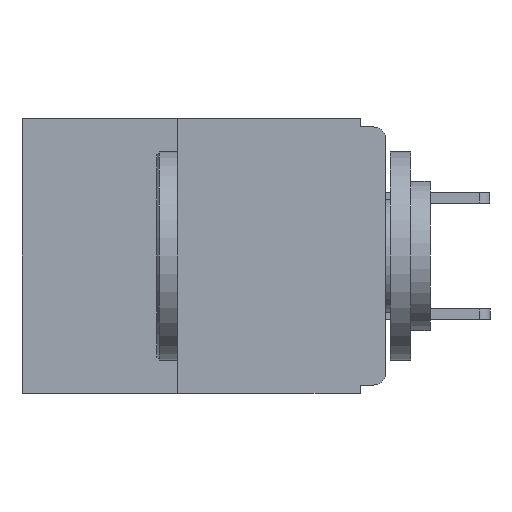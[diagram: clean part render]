
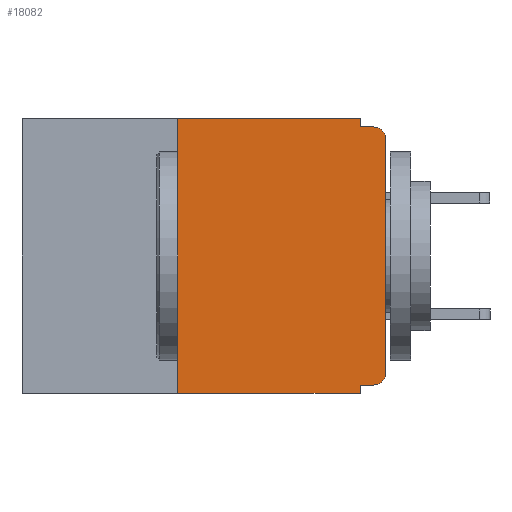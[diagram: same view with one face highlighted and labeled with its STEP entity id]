
A CAD part, left-side view. The second image highlights one B-rep face of the part: STEP entity #18082.
In plain terms, the highlighted planar face has unit normal (-1, 0, 0).
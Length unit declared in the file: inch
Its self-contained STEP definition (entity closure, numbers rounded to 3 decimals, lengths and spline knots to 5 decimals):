
#1279 = VERTEX_POINT ( 'NONE', #4539 ) ;
#1615 = DIRECTION ( 'NONE',  ( 0., 0., -1. ) ) ;
#1627 = AXIS2_PLACEMENT_3D ( 'NONE', #28823, #14491, #31188 ) ;
#1964 = EDGE_CURVE ( 'NONE', #20621, #14345, #23532, .T. ) ;
#3855 = VECTOR ( 'NONE', #27006, 39.37008 ) ;
#4539 = CARTESIAN_POINT ( 'NONE',  ( 0., 0.031, -0.32 ) ) ;
#4628 = DIRECTION ( 'NONE',  ( 0., 1., 0. ) ) ;
#4742 = CARTESIAN_POINT ( 'NONE',  ( 0., 0., -0.32 ) ) ;
#4743 = EDGE_CURVE ( 'NONE', #6605, #1279, #22581, .T. ) ;
#5766 = CARTESIAN_POINT ( 'NONE',  ( 0., 0.437, -0.33 ) ) ;
#5792 = VERTEX_POINT ( 'NONE', #30794 ) ;
#6011 = EDGE_CURVE ( 'NONE', #9688, #10685, #11187, .T. ) ;
#6605 = VERTEX_POINT ( 'NONE', #19673 ) ;
#6651 = DIRECTION ( 'NONE',  ( 0., 0., -1. ) ) ;
#6669 = CIRCLE ( 'NONE', #23854, 0.015 ) ;
#6970 = LINE ( 'NONE', #5766, #31062 ) ;
#7054 = CARTESIAN_POINT ( 'NONE',  ( 0., 0.015, -0.305 ) ) ;
#7147 = ORIENTED_EDGE ( 'NONE', *, *, #6011, .F. ) ;
#7919 = ORIENTED_EDGE ( 'NONE', *, *, #16331, .T. ) ;
#8167 = ORIENTED_EDGE ( 'NONE', *, *, #14884, .T. ) ;
#8579 = ORIENTED_EDGE ( 'NONE', *, *, #21228, .T. ) ;
#8981 = VECTOR ( 'NONE', #4628, 39.37008 ) ;
#9004 = CARTESIAN_POINT ( 'NONE',  ( 0., 0., 0. ) ) ;
#9572 = DIRECTION ( 'NONE',  ( 0., 0., -1. ) ) ;
#9688 = VERTEX_POINT ( 'NONE', #27475 ) ;
#10685 = VERTEX_POINT ( 'NONE', #12097 ) ;
#11022 = EDGE_CURVE ( 'NONE', #5792, #10685, #27361, .T. ) ;
#11187 = LINE ( 'NONE', #27444, #3855 ) ;
#11451 = VECTOR ( 'NONE', #17022, 39.37008 ) ;
#12097 = CARTESIAN_POINT ( 'NONE',  ( 0., 0.015, -0.01 ) ) ;
#12855 = LINE ( 'NONE', #25649, #31166 ) ;
#12887 = CARTESIAN_POINT ( 'NONE',  ( 0., 0.25, -0.33 ) ) ;
#13094 = ORIENTED_EDGE ( 'NONE', *, *, #11022, .T. ) ;
#13636 = ORIENTED_EDGE ( 'NONE', *, *, #20068, .F. ) ;
#14345 = VERTEX_POINT ( 'NONE', #25768 ) ;
#14491 = DIRECTION ( 'NONE',  ( 1., 0., 0. ) ) ;
#14884 = EDGE_CURVE ( 'NONE', #30475, #5792, #18552, .T. ) ;
#14988 = ORIENTED_EDGE ( 'NONE', *, *, #1964, .F. ) ;
#15001 = ORIENTED_EDGE ( 'NONE', *, *, #20771, .F. ) ;
#16298 = DIRECTION ( 'NONE',  ( -1., 0., 0. ) ) ;
#16305 = DIRECTION ( 'NONE',  ( 0., 0., 1. ) ) ;
#16331 = EDGE_CURVE ( 'NONE', #6605, #30475, #6669, .T. ) ;
#16657 = ORIENTED_EDGE ( 'NONE', *, *, #4743, .F. ) ;
#17022 = DIRECTION ( 'NONE',  ( 0., 0., 1. ) ) ;
#17864 = DIRECTION ( 'NONE',  ( 0., -1., 0. ) ) ;
#18082 = ADVANCED_FACE ( 'NONE', ( #30655 ), #24073, .F. ) ;
#18432 = DIRECTION ( 'NONE',  ( 0., 0., -1. ) ) ;
#18552 = LINE ( 'NONE', #9004, #31232 ) ;
#19499 = AXIS2_PLACEMENT_3D ( 'NONE', #30599, #16298, #1615 ) ;
#19673 = CARTESIAN_POINT ( 'NONE',  ( 0., 0.015, -0.32 ) ) ;
#20068 = EDGE_CURVE ( 'NONE', #14345, #23325, #30042, .T. ) ;
#20621 = VERTEX_POINT ( 'NONE', #12887 ) ;
#20771 = EDGE_CURVE ( 'NONE', #23325, #9688, #24811, .T. ) ;
#20801 = CARTESIAN_POINT ( 'NONE',  ( 0., 0.031, 0. ) ) ;
#21173 = CARTESIAN_POINT ( 'NONE',  ( 0., 0., -0.305 ) ) ;
#21201 = CARTESIAN_POINT ( 'NONE',  ( 0., 0.031, 0. ) ) ;
#21228 = EDGE_CURVE ( 'NONE', #20621, #21915, #6970, .T. ) ;
#21915 = VERTEX_POINT ( 'NONE', #25399 ) ;
#22581 = LINE ( 'NONE', #4742, #8981 ) ;
#22704 = CARTESIAN_POINT ( 'NONE',  ( 0., 0.437, 0. ) ) ;
#23325 = VERTEX_POINT ( 'NONE', #20801 ) ;
#23532 = LINE ( 'NONE', #27704, #11451 ) ;
#23744 = VECTOR ( 'NONE', #17864, 39.37008 ) ;
#23854 = AXIS2_PLACEMENT_3D ( 'NONE', #7054, #24025, #9572 ) ;
#24025 = DIRECTION ( 'NONE',  ( -1., 0., 0. ) ) ;
#24073 = PLANE ( 'NONE',  #1627 ) ;
#24811 = LINE ( 'NONE', #21201, #31094 ) ;
#24995 = ORIENTED_EDGE ( 'NONE', *, *, #30414, .F. ) ;
#25399 = CARTESIAN_POINT ( 'NONE',  ( 0., 0.031, -0.33 ) ) ;
#25649 = CARTESIAN_POINT ( 'NONE',  ( 0., 0.031, -0.33 ) ) ;
#25768 = CARTESIAN_POINT ( 'NONE',  ( 0., 0.25, 0. ) ) ;
#27006 = DIRECTION ( 'NONE',  ( 0., -1., 0. ) ) ;
#27361 = CIRCLE ( 'NONE', #19499, 0.015 ) ;
#27444 = CARTESIAN_POINT ( 'NONE',  ( 0., 0., -0.01 ) ) ;
#27475 = CARTESIAN_POINT ( 'NONE',  ( 0., 0.031, -0.01 ) ) ;
#27533 = DIRECTION ( 'NONE',  ( 0., -1., 0. ) ) ;
#27704 = CARTESIAN_POINT ( 'NONE',  ( 0., 0.25, -0.33 ) ) ;
#28823 = CARTESIAN_POINT ( 'NONE',  ( 0., 0.437, 0. ) ) ;
#29026 = EDGE_LOOP ( 'NONE', ( #8167, #13094, #7147, #15001, #13636, #14988, #8579, #24995, #16657, #7919 ) ) ;
#30042 = LINE ( 'NONE', #22704, #23744 ) ;
#30414 = EDGE_CURVE ( 'NONE', #1279, #21915, #12855, .T. ) ;
#30475 = VERTEX_POINT ( 'NONE', #21173 ) ;
#30599 = CARTESIAN_POINT ( 'NONE',  ( 0., 0.015, -0.025 ) ) ;
#30655 = FACE_OUTER_BOUND ( 'NONE', #29026, .T. ) ;
#30794 = CARTESIAN_POINT ( 'NONE',  ( 0., 0., -0.025 ) ) ;
#31062 = VECTOR ( 'NONE', #27533, 39.37008 ) ;
#31094 = VECTOR ( 'NONE', #6651, 39.37008 ) ;
#31166 = VECTOR ( 'NONE', #18432, 39.37008 ) ;
#31188 = DIRECTION ( 'NONE',  ( 0., 0., -1. ) ) ;
#31232 = VECTOR ( 'NONE', #16305, 39.37008 ) ;
